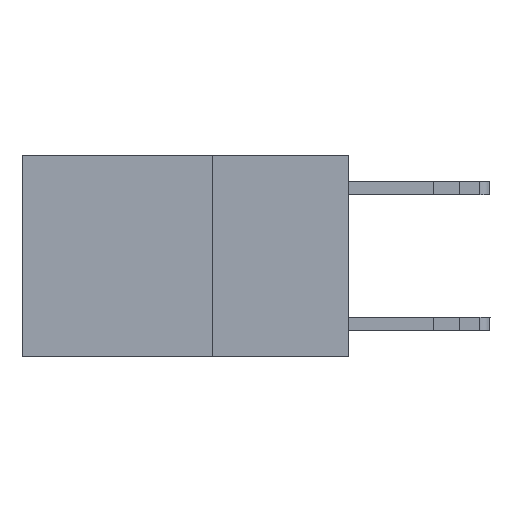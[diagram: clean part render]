
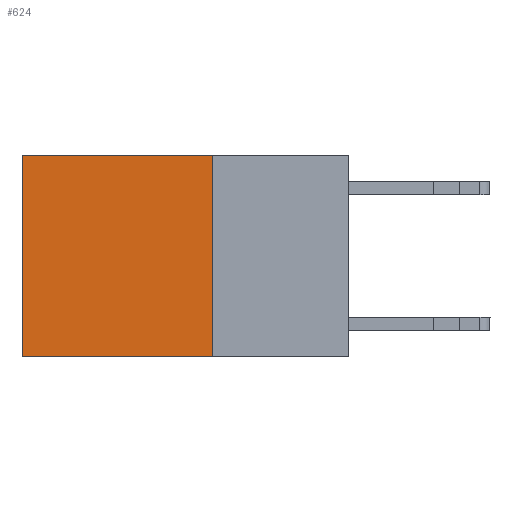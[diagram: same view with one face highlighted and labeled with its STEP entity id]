
A CAD part, left-side view. The second image highlights one B-rep face of the part: STEP entity #624.
In plain terms, the highlighted planar face has unit normal (-1, 0, 0).
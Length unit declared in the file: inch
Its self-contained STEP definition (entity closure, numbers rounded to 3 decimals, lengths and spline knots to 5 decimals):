
#359 = VERTEX_POINT ( 'NONE', #10328 ) ;
#432 = CARTESIAN_POINT ( 'NONE',  ( 0.2625, 0.25, -0.37 ) ) ;
#624 = ADVANCED_FACE ( 'NONE', ( #784 ), #11120, .F. ) ;
#784 = FACE_OUTER_BOUND ( 'NONE', #8013, .T. ) ;
#1423 = LINE ( 'NONE', #20544, #1620 ) ;
#1620 = VECTOR ( 'NONE', #20387, 39.37008 ) ;
#2408 = CARTESIAN_POINT ( 'NONE',  ( 0.2625, 0.6, 0. ) ) ;
#2727 = AXIS2_PLACEMENT_3D ( 'NONE', #13012, #10749, #9597 ) ;
#2755 = EDGE_CURVE ( 'NONE', #18224, #12085, #1423, .T. ) ;
#6999 = VECTOR ( 'NONE', #14536, 39.37008 ) ;
#7049 = LINE ( 'NONE', #15926, #6999 ) ;
#7834 = EDGE_CURVE ( 'NONE', #359, #20552, #7049, .T. ) ;
#8013 = EDGE_LOOP ( 'NONE', ( #20725, #8328, #20098, #19091 ) ) ;
#8328 = ORIENTED_EDGE ( 'NONE', *, *, #2755, .F. ) ;
#8789 = LINE ( 'NONE', #9152, #9281 ) ;
#9152 = CARTESIAN_POINT ( 'NONE',  ( 0.2625, 0.25, 0. ) ) ;
#9281 = VECTOR ( 'NONE', #18752, 39.37008 ) ;
#9597 = DIRECTION ( 'NONE',  ( 0., 0., -1. ) ) ;
#10328 = CARTESIAN_POINT ( 'NONE',  ( 0.2625, 0.25, 0. ) ) ;
#10749 = DIRECTION ( 'NONE',  ( 1., 0., 0. ) ) ;
#11120 = PLANE ( 'NONE',  #2727 ) ;
#12085 = VERTEX_POINT ( 'NONE', #16638 ) ;
#13012 = CARTESIAN_POINT ( 'NONE',  ( 0.2625, 0.25, 0. ) ) ;
#14536 = DIRECTION ( 'NONE',  ( 0., 1., 0. ) ) ;
#15662 = DIRECTION ( 'NONE',  ( 0., 0., -1. ) ) ;
#15694 = CARTESIAN_POINT ( 'NONE',  ( 0.2625, 0.6, 0. ) ) ;
#15926 = CARTESIAN_POINT ( 'NONE',  ( 0.2625, 0.25, 0. ) ) ;
#16638 = CARTESIAN_POINT ( 'NONE',  ( 0.2625, 0.6, -0.37 ) ) ;
#17258 = EDGE_CURVE ( 'NONE', #20552, #12085, #19768, .T. ) ;
#18224 = VERTEX_POINT ( 'NONE', #432 ) ;
#18752 = DIRECTION ( 'NONE',  ( 0., 0., -1. ) ) ;
#19091 = ORIENTED_EDGE ( 'NONE', *, *, #7834, .T. ) ;
#19293 = EDGE_CURVE ( 'NONE', #359, #18224, #8789, .T. ) ;
#19668 = VECTOR ( 'NONE', #15662, 39.37008 ) ;
#19768 = LINE ( 'NONE', #15694, #19668 ) ;
#20098 = ORIENTED_EDGE ( 'NONE', *, *, #19293, .F. ) ;
#20387 = DIRECTION ( 'NONE',  ( 0., 1., 0. ) ) ;
#20544 = CARTESIAN_POINT ( 'NONE',  ( 0.2625, 0.25, -0.37 ) ) ;
#20552 = VERTEX_POINT ( 'NONE', #2408 ) ;
#20725 = ORIENTED_EDGE ( 'NONE', *, *, #17258, .T. ) ;
